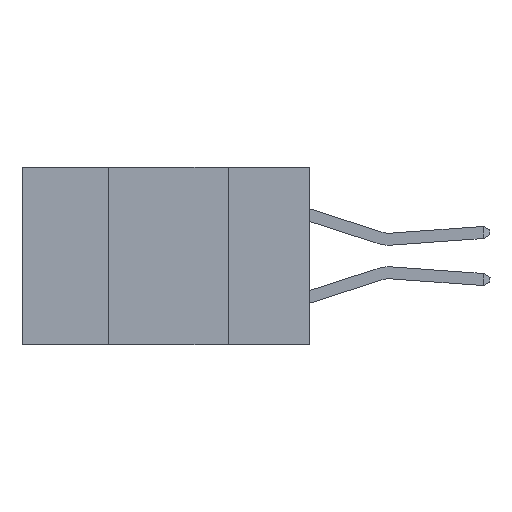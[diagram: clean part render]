
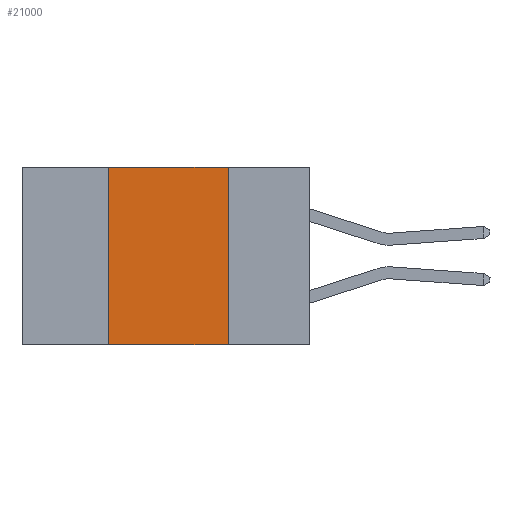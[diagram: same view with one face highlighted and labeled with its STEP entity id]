
A CAD part, left-side view. The second image highlights one B-rep face of the part: STEP entity #21000.
In plain terms, the highlighted planar face has unit normal (-1, 0, 0).
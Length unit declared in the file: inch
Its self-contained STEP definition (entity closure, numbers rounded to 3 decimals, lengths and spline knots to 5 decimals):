
#102 = VERTEX_POINT ( 'NONE', #1298 ) ;
#287 = AXIS2_PLACEMENT_3D ( 'NONE', #9955, #5293, #16518 ) ;
#1298 = CARTESIAN_POINT ( 'NONE',  ( 0., 0.42, 0. ) ) ;
#2772 = DIRECTION ( 'NONE',  ( 0., 0., 1. ) ) ;
#3580 = CARTESIAN_POINT ( 'NONE',  ( 0., 0.17, 0. ) ) ;
#4064 = LINE ( 'NONE', #21741, #27536 ) ;
#4928 = LINE ( 'NONE', #21625, #26654 ) ;
#5293 = DIRECTION ( 'NONE',  ( 1., 0., 0. ) ) ;
#5649 = DIRECTION ( 'NONE',  ( 0., 0., -1. ) ) ;
#6058 = ORIENTED_EDGE ( 'NONE', *, *, #26483, .F. ) ;
#7256 = CARTESIAN_POINT ( 'NONE',  ( 0., 0.17, 0. ) ) ;
#8104 = VECTOR ( 'NONE', #5649, 39.37008 ) ;
#9188 = EDGE_CURVE ( 'NONE', #102, #19002, #4928, .T. ) ;
#9955 = CARTESIAN_POINT ( 'NONE',  ( 0., 0.6, 0. ) ) ;
#10628 = CARTESIAN_POINT ( 'NONE',  ( 0., 0.42, -0.37 ) ) ;
#14135 = LINE ( 'NONE', #3580, #8104 ) ;
#14233 = PLANE ( 'NONE',  #287 ) ;
#15711 = DIRECTION ( 'NONE',  ( 0., -1., 0. ) ) ;
#16518 = DIRECTION ( 'NONE',  ( 0., 0., -1. ) ) ;
#16902 = ORIENTED_EDGE ( 'NONE', *, *, #23667, .F. ) ;
#17722 = ORIENTED_EDGE ( 'NONE', *, *, #9188, .F. ) ;
#17989 = VECTOR ( 'NONE', #15711, 39.37008 ) ;
#19002 = VERTEX_POINT ( 'NONE', #7256 ) ;
#19147 = CARTESIAN_POINT ( 'NONE',  ( 0., 0.17, -0.37 ) ) ;
#19495 = EDGE_LOOP ( 'NONE', ( #16902, #17722, #6058, #25628 ) ) ;
#21000 = ADVANCED_FACE ( 'NONE', ( #28154 ), #14233, .F. ) ;
#21625 = CARTESIAN_POINT ( 'NONE',  ( 0., 0.6, 0. ) ) ;
#21741 = CARTESIAN_POINT ( 'NONE',  ( 0., 0.42, 0. ) ) ;
#22945 = LINE ( 'NONE', #26778, #17989 ) ;
#23531 = VERTEX_POINT ( 'NONE', #19147 ) ;
#23667 = EDGE_CURVE ( 'NONE', #19002, #23531, #14135, .T. ) ;
#25275 = EDGE_CURVE ( 'NONE', #26137, #23531, #22945, .T. ) ;
#25628 = ORIENTED_EDGE ( 'NONE', *, *, #25275, .T. ) ;
#26137 = VERTEX_POINT ( 'NONE', #10628 ) ;
#26483 = EDGE_CURVE ( 'NONE', #26137, #102, #4064, .T. ) ;
#26654 = VECTOR ( 'NONE', #28629, 39.37008 ) ;
#26778 = CARTESIAN_POINT ( 'NONE',  ( 0., 0.6, -0.37 ) ) ;
#27536 = VECTOR ( 'NONE', #2772, 39.37008 ) ;
#28154 = FACE_OUTER_BOUND ( 'NONE', #19495, .T. ) ;
#28629 = DIRECTION ( 'NONE',  ( 0., -1., 0. ) ) ;
